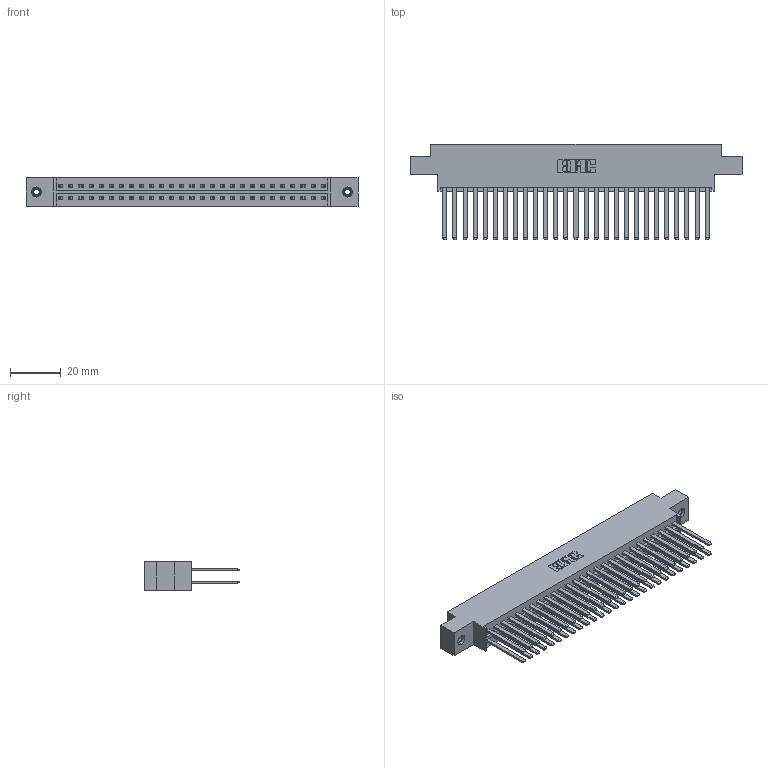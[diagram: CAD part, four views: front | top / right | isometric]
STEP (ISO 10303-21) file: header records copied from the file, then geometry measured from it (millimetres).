
FILE_DESCRIPTION (( 'STEP AP203' ), '1' );
FILE_NAME ('336-054-541-808.STEP', '2020-08-08T00:23:01', ( '' ), ( '' ), 'SwSTEP 2.0', 'SolidWorks 2020', '' );
FILE_SCHEMA (( 'CONFIG_CONTROL_DESIGN' ));
Length unit declared in the file: inch
Products named in the file (4): 336-054-541-808; 345-250-001_345-250-003-102; 336-290-001_336-290-541; 336 Part_Offset - .156 Dia - TI
Assembly tree (57 placements, depth 2):
  336-054-541-808
    336 Part_Offset - .156 Dia - TI
    336-290-001_336-290-541  x54
    345-250-001_345-250-003-102  x2
Bounding box: 130.38 x 37.34 x 11.1 mm (x, y, z)
Volume: 19650.5 mm3; surface area: 24950.9 mm2
Topology: 57 solids, 57 shells, 2446 faces, 7317 edges, 4834 vertices
Faces by surface type: plane 1510, cylinder 920, cone 12, torus 4
Entity records: 23911 total; most frequent: CARTESIAN_POINT 4104, ORIENTED_EDGE 3934, DIRECTION 3453, EDGE_CURVE 1967, VECTOR 1815, LINE 1815, VERTEX_POINT 1306, AXIS2_PLACEMENT_3D 819
